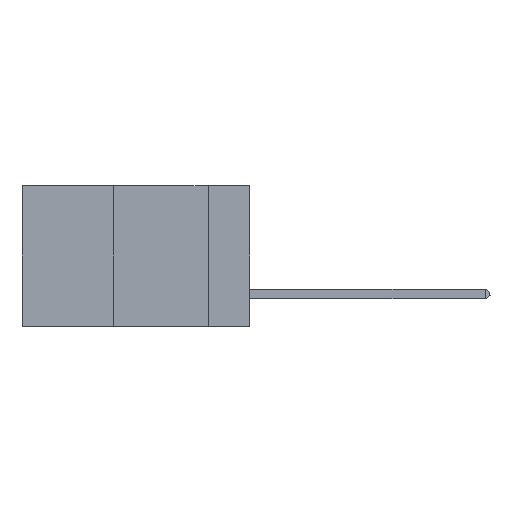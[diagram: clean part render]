
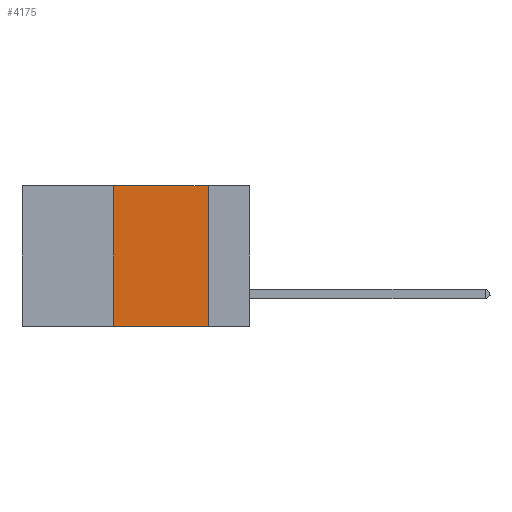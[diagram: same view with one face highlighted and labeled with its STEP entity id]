
A CAD part, left-side view. The second image highlights one B-rep face of the part: STEP entity #4175.
In plain terms, the highlighted planar face has unit normal (-1, 0, 0).
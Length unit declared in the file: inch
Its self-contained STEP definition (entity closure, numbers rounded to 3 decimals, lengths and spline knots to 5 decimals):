
#388 = VECTOR ( 'NONE', #4125, 39.37008 ) ;
#684 = VERTEX_POINT ( 'NONE', #3648 ) ;
#720 = CARTESIAN_POINT ( 'NONE',  ( 0., 0.36, 0. ) ) ;
#1078 = VECTOR ( 'NONE', #3323, 39.37008 ) ;
#1351 = EDGE_CURVE ( 'NONE', #7654, #4908, #7928, .T. ) ;
#2022 = FACE_OUTER_BOUND ( 'NONE', #8558, .T. ) ;
#3205 = PLANE ( 'NONE',  #3883 ) ;
#3323 = DIRECTION ( 'NONE',  ( 0., 0., -1. ) ) ;
#3616 = VECTOR ( 'NONE', #10598, 39.37008 ) ;
#3648 = CARTESIAN_POINT ( 'NONE',  ( 0., 0.11, 0. ) ) ;
#3883 = AXIS2_PLACEMENT_3D ( 'NONE', #10553, #7360, #5643 ) ;
#3885 = CARTESIAN_POINT ( 'NONE',  ( 0., 0.36, -0.37 ) ) ;
#3927 = ORIENTED_EDGE ( 'NONE', *, *, #6668, .F. ) ;
#3968 = ORIENTED_EDGE ( 'NONE', *, *, #5596, .F. ) ;
#4125 = DIRECTION ( 'NONE',  ( 0., -1., 0. ) ) ;
#4175 = ADVANCED_FACE ( 'NONE', ( #2022 ), #3205, .F. ) ;
#4615 = DIRECTION ( 'NONE',  ( 0., -1., 0. ) ) ;
#4908 = VERTEX_POINT ( 'NONE', #5269 ) ;
#5269 = CARTESIAN_POINT ( 'NONE',  ( 0., 0.11, -0.37 ) ) ;
#5596 = EDGE_CURVE ( 'NONE', #6208, #684, #6788, .T. ) ;
#5643 = DIRECTION ( 'NONE',  ( 0., 0., -1. ) ) ;
#5719 = CARTESIAN_POINT ( 'NONE',  ( 0., 0.36, 0. ) ) ;
#5784 = LINE ( 'NONE', #5719, #3616 ) ;
#6208 = VERTEX_POINT ( 'NONE', #720 ) ;
#6384 = ORIENTED_EDGE ( 'NONE', *, *, #8036, .F. ) ;
#6517 = VECTOR ( 'NONE', #4615, 39.37008 ) ;
#6616 = CARTESIAN_POINT ( 'NONE',  ( 0., 0.6, -0.37 ) ) ;
#6668 = EDGE_CURVE ( 'NONE', #7654, #6208, #5784, .T. ) ;
#6788 = LINE ( 'NONE', #8823, #6517 ) ;
#7360 = DIRECTION ( 'NONE',  ( 1., 0., 0. ) ) ;
#7654 = VERTEX_POINT ( 'NONE', #3885 ) ;
#7850 = LINE ( 'NONE', #8170, #1078 ) ;
#7928 = LINE ( 'NONE', #6616, #388 ) ;
#8036 = EDGE_CURVE ( 'NONE', #684, #4908, #7850, .T. ) ;
#8170 = CARTESIAN_POINT ( 'NONE',  ( 0., 0.11, 0. ) ) ;
#8558 = EDGE_LOOP ( 'NONE', ( #6384, #3968, #3927, #10637 ) ) ;
#8823 = CARTESIAN_POINT ( 'NONE',  ( 0., 0.6, 0. ) ) ;
#10553 = CARTESIAN_POINT ( 'NONE',  ( 0., 0.6, 0. ) ) ;
#10598 = DIRECTION ( 'NONE',  ( 0., 0., 1. ) ) ;
#10637 = ORIENTED_EDGE ( 'NONE', *, *, #1351, .T. ) ;
